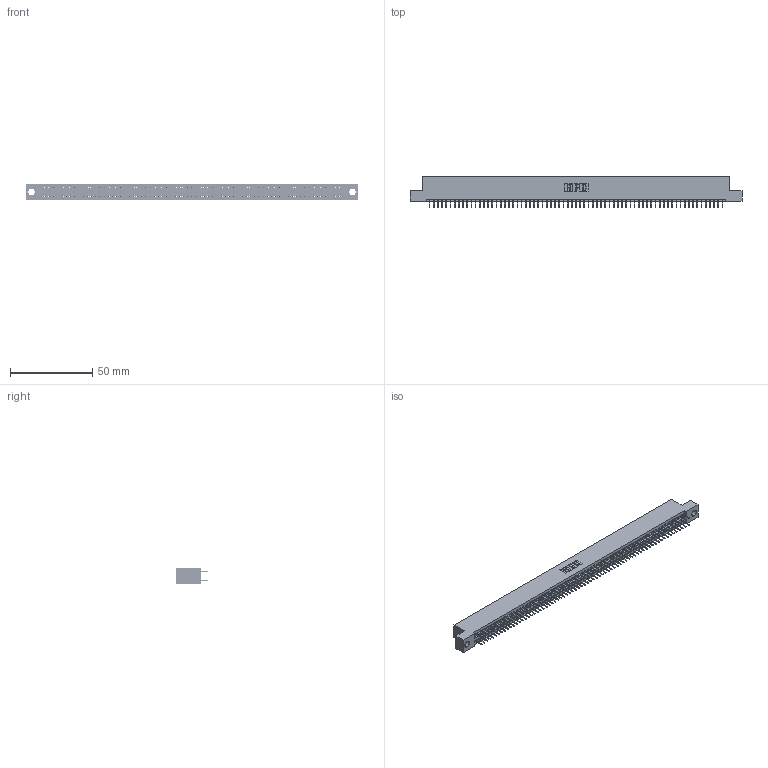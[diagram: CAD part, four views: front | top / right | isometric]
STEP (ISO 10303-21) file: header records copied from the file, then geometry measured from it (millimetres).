
FILE_DESCRIPTION (( 'STEP AP203' ), '1' );
FILE_NAME ('345-142-524-204.STEP', '2021-05-26T01:49:06', ( '' ), ( '' ), 'SwSTEP 2.0', 'SolidWorks 2020', '' );
FILE_SCHEMA (( 'CONFIG_CONTROL_DESIGN' ));
Length unit declared in the file: inch
Products named in the file (3): 345 Part_Flush Mounting Lugs - 0.156 Dia-TI; 345-142-524-204; 345-292-001_345-293-124
Assembly tree (143 placements, depth 2):
  345-142-524-204
    345 Part_Flush Mounting Lugs - 0.156 Dia-TI
    345-292-001_345-293-124  x142
Bounding box: 201.55 x 19.35 x 9.4 mm (x, y, z)
Volume: 19527 mm3; surface area: 28710.2 mm2
Topology: 143 solids, 143 shells, 7808 faces, 22103 edges, 14166 vertices
Faces by surface type: plane 5632, cylinder 2176
Entity records: 52297 total; most frequent: CARTESIAN_POINT 8742, ORIENTED_EDGE 8674, DIRECTION 7673, EDGE_CURVE 4337, LINE 3925, VECTOR 3925, VERTEX_POINT 2886, AXIS2_PLACEMENT_3D 1874
